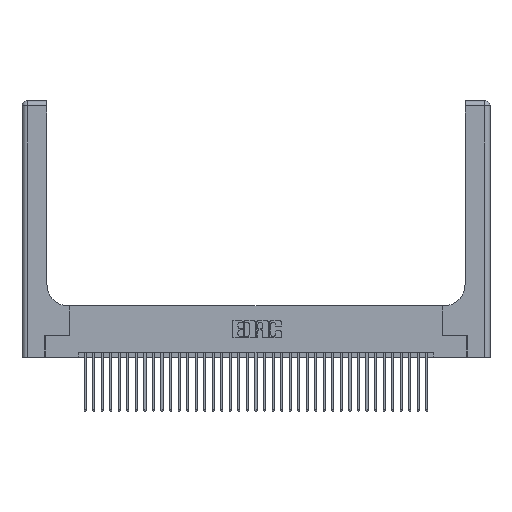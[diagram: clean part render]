
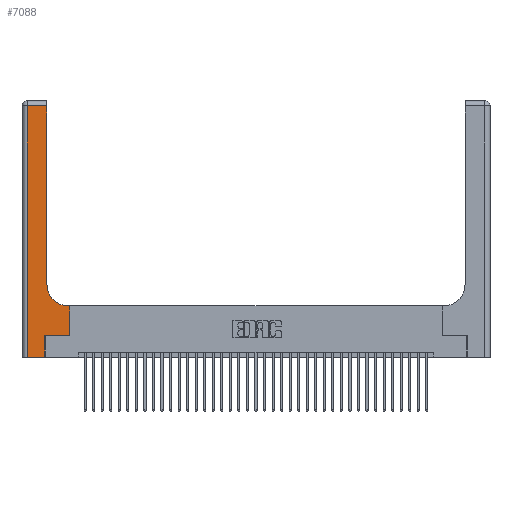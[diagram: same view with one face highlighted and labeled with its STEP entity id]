
A CAD part, top view. The second image highlights one B-rep face of the part: STEP entity #7088.
In plain terms, the highlighted planar face has unit normal (0, 0, 1).
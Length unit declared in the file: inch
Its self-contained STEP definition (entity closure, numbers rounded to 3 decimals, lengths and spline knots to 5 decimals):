
#40 = ORIENTED_EDGE ( 'NONE', *, *, #31179, .T. ) ;
#334 = CARTESIAN_POINT ( 'NONE',  ( 0.2915, 2.94, 0.37 ) ) ;
#1222 = VERTEX_POINT ( 'NONE', #33211 ) ;
#1363 = VECTOR ( 'NONE', #21468, 39.37008 ) ;
#2234 = DIRECTION ( 'NONE',  ( 0., 1., 0. ) ) ;
#2622 = DIRECTION ( 'NONE',  ( -1., 0., 0. ) ) ;
#3048 = AXIS2_PLACEMENT_3D ( 'NONE', #25719, #8370, #28569 ) ;
#4008 = VECTOR ( 'NONE', #11443, 39.37008 ) ;
#6231 = CARTESIAN_POINT ( 'NONE',  ( 0.5415, 0.6, 0.37 ) ) ;
#6307 = CARTESIAN_POINT ( 'NONE',  ( 0., 3., 0.37 ) ) ;
#6993 = VERTEX_POINT ( 'NONE', #26222 ) ;
#7087 = CIRCLE ( 'NONE', #3048, 0.25 ) ;
#7088 = ADVANCED_FACE ( 'NONE', ( #23933 ), #23736, .F. ) ;
#7129 = EDGE_LOOP ( 'NONE', ( #35786, #40, #10727, #16245, #33214, #20706, #12578, #9216, #7241 ) ) ;
#7241 = ORIENTED_EDGE ( 'NONE', *, *, #16303, .T. ) ;
#8370 = DIRECTION ( 'NONE',  ( 0., 0., -1. ) ) ;
#8517 = LINE ( 'NONE', #27779, #30610 ) ;
#9124 = CARTESIAN_POINT ( 'NONE',  ( 0.2915, 0.85, 0.37 ) ) ;
#9216 = ORIENTED_EDGE ( 'NONE', *, *, #28249, .T. ) ;
#9262 = DIRECTION ( 'NONE',  ( 0., 0., -1. ) ) ;
#10727 = ORIENTED_EDGE ( 'NONE', *, *, #24761, .T. ) ;
#11226 = CARTESIAN_POINT ( 'NONE',  ( 0.06, 2.94, 0.37 ) ) ;
#11443 = DIRECTION ( 'NONE',  ( 0., 1., 0. ) ) ;
#12578 = ORIENTED_EDGE ( 'NONE', *, *, #26054, .T. ) ;
#12990 = VECTOR ( 'NONE', #2622, 39.37008 ) ;
#13676 = EDGE_CURVE ( 'NONE', #33847, #34988, #31153, .T. ) ;
#13914 = DIRECTION ( 'NONE',  ( 1., 0., 0. ) ) ;
#14130 = DIRECTION ( 'NONE',  ( -1., 0., 0. ) ) ;
#14861 = EDGE_CURVE ( 'NONE', #1222, #33847, #8517, .T. ) ;
#14993 = VERTEX_POINT ( 'NONE', #11226 ) ;
#16245 = ORIENTED_EDGE ( 'NONE', *, *, #14861, .T. ) ;
#16303 = EDGE_CURVE ( 'NONE', #20430, #32713, #7087, .T. ) ;
#16999 = LINE ( 'NONE', #35445, #1363 ) ;
#18282 = CARTESIAN_POINT ( 'NONE',  ( 0.269, 0.25, 0.37 ) ) ;
#18335 = VECTOR ( 'NONE', #2234, 39.37008 ) ;
#19853 = CARTESIAN_POINT ( 'NONE',  ( 0.2915, 0.6, 0.37 ) ) ;
#20378 = AXIS2_PLACEMENT_3D ( 'NONE', #6307, #9262, #29443 ) ;
#20430 = VERTEX_POINT ( 'NONE', #6231 ) ;
#20680 = VECTOR ( 'NONE', #31139, 39.37008 ) ;
#20706 = ORIENTED_EDGE ( 'NONE', *, *, #26012, .T. ) ;
#20710 = LINE ( 'NONE', #37214, #12990 ) ;
#21005 = VERTEX_POINT ( 'NONE', #334 ) ;
#21468 = DIRECTION ( 'NONE',  ( 0., -1., 0. ) ) ;
#22673 = CARTESIAN_POINT ( 'NONE',  ( 0.5585, 0.25, 0.37 ) ) ;
#23200 = CARTESIAN_POINT ( 'NONE',  ( 0.5585, 0.6, 0.37 ) ) ;
#23722 = EDGE_CURVE ( 'NONE', #32713, #21005, #34979, .T. ) ;
#23736 = PLANE ( 'NONE',  #20378 ) ;
#23933 = FACE_OUTER_BOUND ( 'NONE', #7129, .T. ) ;
#24761 = EDGE_CURVE ( 'NONE', #14993, #1222, #16999, .T. ) ;
#25719 = CARTESIAN_POINT ( 'NONE',  ( 0.5415, 0.85, 0.37 ) ) ;
#25951 = LINE ( 'NONE', #22673, #18335 ) ;
#26012 = EDGE_CURVE ( 'NONE', #34988, #6993, #26834, .T. ) ;
#26054 = EDGE_CURVE ( 'NONE', #6993, #28753, #25951, .T. ) ;
#26222 = CARTESIAN_POINT ( 'NONE',  ( 0.5585, 0.25, 0.37 ) ) ;
#26834 = LINE ( 'NONE', #31132, #34416 ) ;
#27779 = CARTESIAN_POINT ( 'NONE',  ( 0., 0., 0.37 ) ) ;
#28249 = EDGE_CURVE ( 'NONE', #28753, #20430, #29377, .T. ) ;
#28284 = CARTESIAN_POINT ( 'NONE',  ( 0.2915, 3., 0.37 ) ) ;
#28569 = DIRECTION ( 'NONE',  ( 1., 0., 0. ) ) ;
#28753 = VERTEX_POINT ( 'NONE', #23200 ) ;
#29377 = LINE ( 'NONE', #19853, #35182 ) ;
#29443 = DIRECTION ( 'NONE',  ( -1., 0., 0. ) ) ;
#30610 = VECTOR ( 'NONE', #30626, 39.37008 ) ;
#30626 = DIRECTION ( 'NONE',  ( 1., 0., 0. ) ) ;
#31132 = CARTESIAN_POINT ( 'NONE',  ( 0.269, 0.25, 0.37 ) ) ;
#31139 = DIRECTION ( 'NONE',  ( 0., 1., 0. ) ) ;
#31153 = LINE ( 'NONE', #31580, #4008 ) ;
#31179 = EDGE_CURVE ( 'NONE', #21005, #14993, #20710, .T. ) ;
#31580 = CARTESIAN_POINT ( 'NONE',  ( 0.269, 0., 0.37 ) ) ;
#32713 = VERTEX_POINT ( 'NONE', #9124 ) ;
#33211 = CARTESIAN_POINT ( 'NONE',  ( 0.06, 0., 0.37 ) ) ;
#33214 = ORIENTED_EDGE ( 'NONE', *, *, #13676, .T. ) ;
#33847 = VERTEX_POINT ( 'NONE', #34716 ) ;
#34416 = VECTOR ( 'NONE', #13914, 39.37008 ) ;
#34716 = CARTESIAN_POINT ( 'NONE',  ( 0.269, 0., 0.37 ) ) ;
#34979 = LINE ( 'NONE', #28284, #20680 ) ;
#34988 = VERTEX_POINT ( 'NONE', #18282 ) ;
#35182 = VECTOR ( 'NONE', #14130, 39.37008 ) ;
#35445 = CARTESIAN_POINT ( 'NONE',  ( 0.06, 3., 0.37 ) ) ;
#35786 = ORIENTED_EDGE ( 'NONE', *, *, #23722, .T. ) ;
#37214 = CARTESIAN_POINT ( 'NONE',  ( 0., 2.94, 0.37 ) ) ;
